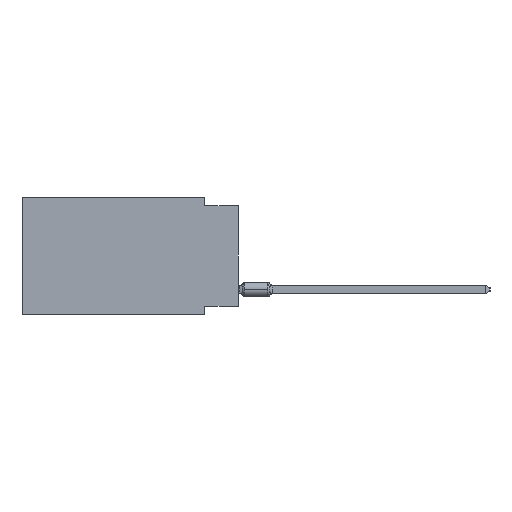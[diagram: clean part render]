
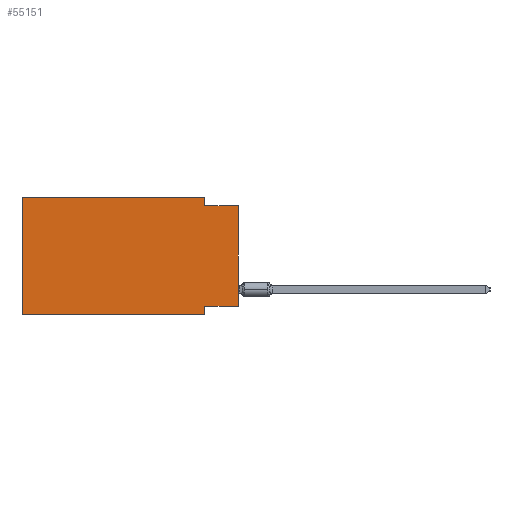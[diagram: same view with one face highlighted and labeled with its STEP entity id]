
A CAD part, left-side view. The second image highlights one B-rep face of the part: STEP entity #55151.
In plain terms, the highlighted planar face has unit normal (-1, 0, 0).
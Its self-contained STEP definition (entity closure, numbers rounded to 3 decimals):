
#675 = DIRECTION ( 'NONE',  ( 0., 0., 1. ) ) ;
#1300 = EDGE_CURVE ( 'NONE', #3274, #18713, #42435, .T. ) ;
#3274 = VERTEX_POINT ( 'NONE', #11986 ) ;
#4345 = VECTOR ( 'NONE', #56668, 1000. ) ;
#7033 = VECTOR ( 'NONE', #50832, 1000. ) ;
#8526 = VERTEX_POINT ( 'NONE', #78262 ) ;
#8900 = LINE ( 'NONE', #24023, #62742 ) ;
#8915 = CARTESIAN_POINT ( 'NONE',  ( 0., 2.54, -8.89 ) ) ;
#8954 = ORIENTED_EDGE ( 'NONE', *, *, #31641, .F. ) ;
#9157 = CARTESIAN_POINT ( 'NONE',  ( 0., 16.383, 0. ) ) ;
#9175 = FACE_OUTER_BOUND ( 'NONE', #70091, .T. ) ;
#10316 = CARTESIAN_POINT ( 'NONE',  ( 0., 16.383, 0. ) ) ;
#10727 = ORIENTED_EDGE ( 'NONE', *, *, #47659, .T. ) ;
#11986 = CARTESIAN_POINT ( 'NONE',  ( 0., 0., -8.255 ) ) ;
#13941 = CARTESIAN_POINT ( 'NONE',  ( 0., 2.54, -8.89 ) ) ;
#15823 = CARTESIAN_POINT ( 'NONE',  ( 0., 16.383, 0. ) ) ;
#16228 = VERTEX_POINT ( 'NONE', #8915 ) ;
#18713 = VERTEX_POINT ( 'NONE', #19288 ) ;
#19241 = CARTESIAN_POINT ( 'NONE',  ( 0., 2.54, -0.635 ) ) ;
#19288 = CARTESIAN_POINT ( 'NONE',  ( 0., 2.54, -8.255 ) ) ;
#22418 = LINE ( 'NONE', #13941, #7033 ) ;
#23425 = DIRECTION ( 'NONE',  ( 0., -1., 0. ) ) ;
#24023 = CARTESIAN_POINT ( 'NONE',  ( 0., 2.54, 0. ) ) ;
#24738 = VERTEX_POINT ( 'NONE', #84002 ) ;
#26175 = EDGE_CURVE ( 'NONE', #24738, #77373, #73987, .T. ) ;
#27601 = LINE ( 'NONE', #83963, #46068 ) ;
#31641 = EDGE_CURVE ( 'NONE', #18713, #16228, #22418, .T. ) ;
#32959 = ORIENTED_EDGE ( 'NONE', *, *, #51388, .T. ) ;
#36270 = CARTESIAN_POINT ( 'NONE',  ( 0., 0., 0. ) ) ;
#36376 = VECTOR ( 'NONE', #23425, 1000. ) ;
#36640 = DIRECTION ( 'NONE',  ( 0., 0., -1. ) ) ;
#36831 = VECTOR ( 'NONE', #675, 1000. ) ;
#37634 = CARTESIAN_POINT ( 'NONE',  ( 0., 0., -0.635 ) ) ;
#37772 = DIRECTION ( 'NONE',  ( 0., 0., -1. ) ) ;
#40703 = VERTEX_POINT ( 'NONE', #84530 ) ;
#41483 = ORIENTED_EDGE ( 'NONE', *, *, #82931, .F. ) ;
#42435 = LINE ( 'NONE', #71296, #4345 ) ;
#43737 = PLANE ( 'NONE',  #61609 ) ;
#46068 = VECTOR ( 'NONE', #47537, 1000. ) ;
#47537 = DIRECTION ( 'NONE',  ( 0., -1., 0. ) ) ;
#47659 = EDGE_CURVE ( 'NONE', #24738, #16228, #27601, .T. ) ;
#48928 = VERTEX_POINT ( 'NONE', #19241 ) ;
#49976 = EDGE_CURVE ( 'NONE', #40703, #48928, #8900, .T. ) ;
#50832 = DIRECTION ( 'NONE',  ( 0., 0., -1. ) ) ;
#51388 = EDGE_CURVE ( 'NONE', #3274, #8526, #71297, .T. ) ;
#55151 = ADVANCED_FACE ( 'NONE', ( #9175 ), #43737, .F. ) ;
#55772 = ORIENTED_EDGE ( 'NONE', *, *, #49976, .F. ) ;
#55979 = VECTOR ( 'NONE', #85943, 1000. ) ;
#56668 = DIRECTION ( 'NONE',  ( 0., 1., 0. ) ) ;
#57096 = CARTESIAN_POINT ( 'NONE',  ( 0., 16.383, 0. ) ) ;
#59875 = LINE ( 'NONE', #37634, #36376 ) ;
#60311 = EDGE_CURVE ( 'NONE', #48928, #8526, #59875, .T. ) ;
#61609 = AXIS2_PLACEMENT_3D ( 'NONE', #15823, #72587, #36640 ) ;
#62742 = VECTOR ( 'NONE', #37772, 1000. ) ;
#70091 = EDGE_LOOP ( 'NONE', ( #32959, #70518, #55772, #41483, #88731, #10727, #8954, #81752 ) ) ;
#70518 = ORIENTED_EDGE ( 'NONE', *, *, #60311, .F. ) ;
#71296 = CARTESIAN_POINT ( 'NONE',  ( 0., 0., -8.255 ) ) ;
#71297 = LINE ( 'NONE', #36270, #74359 ) ;
#72587 = DIRECTION ( 'NONE',  ( 1., 0., 0. ) ) ;
#73987 = LINE ( 'NONE', #9157, #36831 ) ;
#74359 = VECTOR ( 'NONE', #92609, 1000. ) ;
#77373 = VERTEX_POINT ( 'NONE', #10316 ) ;
#78262 = CARTESIAN_POINT ( 'NONE',  ( 0., 0., -0.635 ) ) ;
#81752 = ORIENTED_EDGE ( 'NONE', *, *, #1300, .F. ) ;
#82931 = EDGE_CURVE ( 'NONE', #77373, #40703, #93507, .T. ) ;
#83963 = CARTESIAN_POINT ( 'NONE',  ( 0., 16.383, -8.89 ) ) ;
#84002 = CARTESIAN_POINT ( 'NONE',  ( 0., 16.383, -8.89 ) ) ;
#84530 = CARTESIAN_POINT ( 'NONE',  ( 0., 2.54, 0. ) ) ;
#85943 = DIRECTION ( 'NONE',  ( 0., -1., 0. ) ) ;
#88731 = ORIENTED_EDGE ( 'NONE', *, *, #26175, .F. ) ;
#92609 = DIRECTION ( 'NONE',  ( 0., 0., 1. ) ) ;
#93507 = LINE ( 'NONE', #57096, #55979 ) ;
